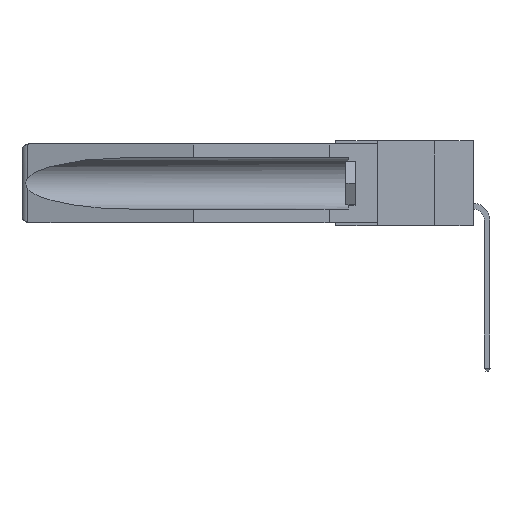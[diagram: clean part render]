
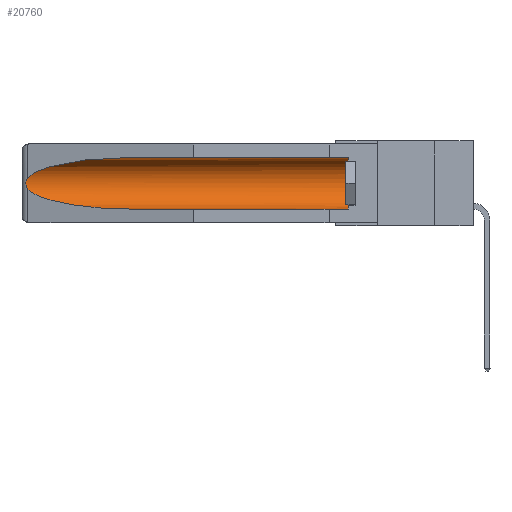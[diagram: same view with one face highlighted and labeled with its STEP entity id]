
A CAD part, left-side view. The second image highlights one B-rep face of the part: STEP entity #20760.
In plain terms, the highlighted cylindrical face has radius 2.857 mm (diameter 5.715 mm), a partial arc.
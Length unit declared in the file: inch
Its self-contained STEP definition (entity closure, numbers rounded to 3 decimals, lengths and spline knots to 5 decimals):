
#669 = CARTESIAN_POINT ( 'NONE',  ( 0.26655, 1.53094, -0.18657 ) ) ;
#2077 = VERTEX_POINT ( 'NONE', #29084 ) ;
#2143 = FACE_OUTER_BOUND ( 'NONE', #22965, .T. ) ;
#2144 = CARTESIAN_POINT ( 'NONE',  ( 0.155, 0.126, -0.1715 ) ) ;
#2425 = EDGE_CURVE ( 'NONE', #2077, #4910, #13472, .T. ) ;
#2569 = ORIENTED_EDGE ( 'NONE', *, *, #2425, .T. ) ;
#3018 = VECTOR ( 'NONE', #15018, 39.37008 ) ;
#3340 = CARTESIAN_POINT ( 'NONE',  ( 0.155, 1.07973, -0.059 ) ) ;
#4267 = ORIENTED_EDGE ( 'NONE', *, *, #22923, .T. ) ;
#4910 = VERTEX_POINT ( 'NONE', #25882 ) ;
#5809 = ORIENTED_EDGE ( 'NONE', *, *, #6729, .T. ) ;
#6066 = ORIENTED_EDGE ( 'NONE', *, *, #20719, .F. ) ;
#6456 = CARTESIAN_POINT ( 'NONE',  ( 0.21114, 1.30732, -0.284 ) ) ;
#6611 = VERTEX_POINT ( 'NONE', #29539 ) ;
#6723 = ORIENTED_EDGE ( 'NONE', *, *, #10376, .T. ) ;
#6729 = EDGE_CURVE ( 'NONE', #26265, #6611, #13954, .T. ) ;
#6982 = B_SPLINE_CURVE_WITH_KNOTS ( 'NONE', 3,
 ( #17633, #8220, #25421, #15554, #30458, #25735, #25635, #669, #13192, #30801 ),
 .UNSPECIFIED., .F., .F.,
 ( 4, 2, 2, 2, 4 ),
 ( 0., 0.00029, 0.00058, 0.00087, 0.00117 ),
 .UNSPECIFIED. ) ;
#8220 = CARTESIAN_POINT ( 'NONE',  ( 0.26597, 1.52961, -0.15275 ) ) ;
#8227 = CARTESIAN_POINT ( 'NONE',  ( 0.155, 1.07973, -0.284 ) ) ;
#8644 = DIRECTION ( 'NONE',  ( 0., 1., 0. ) ) ;
#8665 = CARTESIAN_POINT ( 'NONE',  ( 0.26537, 1.52718, -0.14972 ) ) ;
#8866 = CARTESIAN_POINT ( 'NONE',  ( 0.26537, 1.52718, -0.19328 ) ) ;
#9292 = EDGE_CURVE ( 'NONE', #22924, #12840, #19371, .T. ) ;
#9306 = AXIS2_PLACEMENT_3D ( 'NONE', #2144, #27305, #17027 ) ;
#10376 = EDGE_CURVE ( 'NONE', #6611, #2077, #18898, .T. ) ;
#10757 = CARTESIAN_POINT ( 'NONE',  ( 0.155, -0.30754, -0.1715 ) ) ;
#11089 = CARTESIAN_POINT ( 'NONE',  ( 0.25451, 1.48313, -0.24835 ) ) ;
#11525 = CARTESIAN_POINT ( 'NONE',  ( 0.25451, 1.48313, -0.09465 ) ) ;
#11982 = ORIENTED_EDGE ( 'NONE', *, *, #9292, .T. ) ;
#12840 = VERTEX_POINT ( 'NONE', #8227 ) ;
#13192 = CARTESIAN_POINT ( 'NONE',  ( 0.26597, 1.5296, -0.19026 ) ) ;
#13292 = DIRECTION ( 'NONE',  ( 0., 0., 1. ) ) ;
#13472 =( BOUNDED_CURVE ( )  B_SPLINE_CURVE ( 3, ( #3340, #13865, #11525, #8665 ),
 .UNSPECIFIED., .F., .F. ) 
 B_SPLINE_CURVE_WITH_KNOTS ( ( 4, 4 ),
 ( 4.71239, 6.08839 ),
 .UNSPECIFIED. ) 
 CURVE ( )  GEOMETRIC_REPRESENTATION_ITEM ( )  RATIONAL_B_SPLINE_CURVE ( ( 1., 0.848, 0.848, 1. ) ) 
 REPRESENTATION_ITEM ( '' )  );
#13759 = CARTESIAN_POINT ( 'NONE',  ( 0.155, 1.07973, -0.284 ) ) ;
#13865 = CARTESIAN_POINT ( 'NONE',  ( 0.21114, 1.30732, -0.059 ) ) ;
#13954 = CIRCLE ( 'NONE', #9306, 0.1125 ) ;
#15018 = DIRECTION ( 'NONE',  ( 0., 1., 0. ) ) ;
#15554 = CARTESIAN_POINT ( 'NONE',  ( 0.2673, 1.5327, -0.16383 ) ) ;
#15763 = DIRECTION ( 'NONE',  ( 0., 1., 0. ) ) ;
#16477 = VECTOR ( 'NONE', #8644, 39.37008 ) ;
#17027 = DIRECTION ( 'NONE',  ( 0., 0., 1. ) ) ;
#17633 = CARTESIAN_POINT ( 'NONE',  ( 0.26537, 1.52718, -0.14972 ) ) ;
#18898 = LINE ( 'NONE', #30063, #3018 ) ;
#19371 =( BOUNDED_CURVE ( )  B_SPLINE_CURVE ( 3, ( #8866, #11089, #6456, #13759 ),
 .UNSPECIFIED., .F., .F. ) 
 B_SPLINE_CURVE_WITH_KNOTS ( ( 4, 4 ),
 ( 0.1948, 1.5708 ),
 .UNSPECIFIED. ) 
 CURVE ( )  GEOMETRIC_REPRESENTATION_ITEM ( )  RATIONAL_B_SPLINE_CURVE ( ( 1., 0.848, 0.848, 1. ) ) 
 REPRESENTATION_ITEM ( '' )  );
#20719 = EDGE_CURVE ( 'NONE', #26265, #12840, #26644, .T. ) ;
#20760 = ADVANCED_FACE ( 'NONE', ( #2143 ), #23933, .F. ) ;
#22923 = EDGE_CURVE ( 'NONE', #4910, #22924, #6982, .T. ) ;
#22924 = VERTEX_POINT ( 'NONE', #26951 ) ;
#22965 = EDGE_LOOP ( 'NONE', ( #2569, #4267, #11982, #6066, #5809, #6723 ) ) ;
#23933 = CYLINDRICAL_SURFACE ( 'NONE', #28562, 0.1125 ) ;
#25421 = CARTESIAN_POINT ( 'NONE',  ( 0.26654, 1.53092, -0.15636 ) ) ;
#25635 = CARTESIAN_POINT ( 'NONE',  ( 0.2673, 1.53269, -0.17917 ) ) ;
#25735 = CARTESIAN_POINT ( 'NONE',  ( 0.2675, 1.53308, -0.17534 ) ) ;
#25826 = CARTESIAN_POINT ( 'NONE',  ( 0.155, -0.30754, -0.284 ) ) ;
#25882 = CARTESIAN_POINT ( 'NONE',  ( 0.26537, 1.52718, -0.14972 ) ) ;
#26265 = VERTEX_POINT ( 'NONE', #28374 ) ;
#26644 = LINE ( 'NONE', #25826, #16477 ) ;
#26951 = CARTESIAN_POINT ( 'NONE',  ( 0.26537, 1.52718, -0.19328 ) ) ;
#27305 = DIRECTION ( 'NONE',  ( 0., -1., 0. ) ) ;
#28374 = CARTESIAN_POINT ( 'NONE',  ( 0.155, 0.126, -0.284 ) ) ;
#28562 = AXIS2_PLACEMENT_3D ( 'NONE', #10757, #15763, #13292 ) ;
#29084 = CARTESIAN_POINT ( 'NONE',  ( 0.155, 1.07973, -0.059 ) ) ;
#29539 = CARTESIAN_POINT ( 'NONE',  ( 0.155, 0.126, -0.059 ) ) ;
#30063 = CARTESIAN_POINT ( 'NONE',  ( 0.155, -0.30754, -0.059 ) ) ;
#30458 = CARTESIAN_POINT ( 'NONE',  ( 0.2675, 1.53308, -0.16763 ) ) ;
#30801 = CARTESIAN_POINT ( 'NONE',  ( 0.26537, 1.52718, -0.19328 ) ) ;
